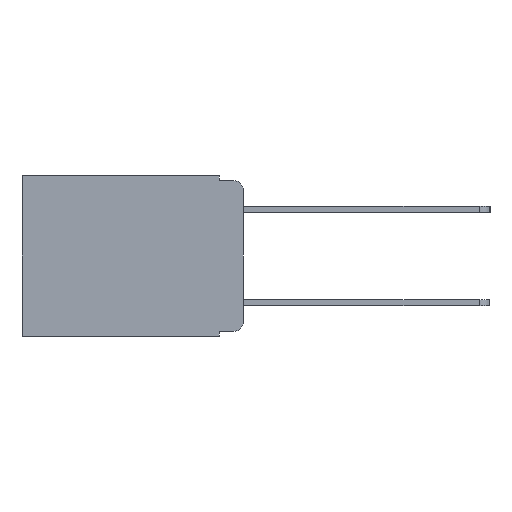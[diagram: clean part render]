
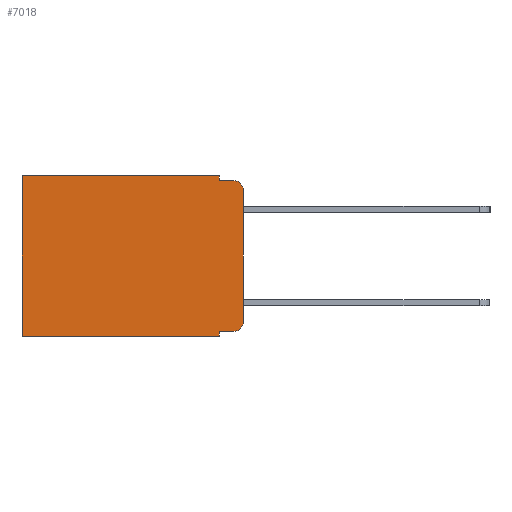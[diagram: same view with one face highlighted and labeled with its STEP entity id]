
A CAD part, left-side view. The second image highlights one B-rep face of the part: STEP entity #7018.
In plain terms, the highlighted planar face has unit normal (-1, 0, 0).
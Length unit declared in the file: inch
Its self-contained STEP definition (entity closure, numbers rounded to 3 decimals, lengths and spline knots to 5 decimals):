
#772 = CARTESIAN_POINT ( 'NONE',  ( 0.298, 0.473, 0. ) ) ;
#1231 = VERTEX_POINT ( 'NONE', #13358 ) ;
#1259 = ORIENTED_EDGE ( 'NONE', *, *, #11092, .T. ) ;
#1486 = DIRECTION ( 'NONE',  ( 0., 0., -1. ) ) ;
#1542 = VERTEX_POINT ( 'NONE', #14407 ) ;
#2212 = VECTOR ( 'NONE', #12062, 39.37008 ) ;
#2250 = VERTEX_POINT ( 'NONE', #7508 ) ;
#2955 = LINE ( 'NONE', #7042, #14989 ) ;
#3022 = CARTESIAN_POINT ( 'NONE',  ( 0.298, 0.02, -0.03 ) ) ;
#3057 = ORIENTED_EDGE ( 'NONE', *, *, #14924, .F. ) ;
#3107 = CARTESIAN_POINT ( 'NONE',  ( 0.298, 0.051, -0.333 ) ) ;
#3242 = CARTESIAN_POINT ( 'NONE',  ( 0.298, 0., -0.03 ) ) ;
#3285 = ORIENTED_EDGE ( 'NONE', *, *, #13959, .F. ) ;
#3559 = LINE ( 'NONE', #6247, #11307 ) ;
#3753 = VERTEX_POINT ( 'NONE', #772 ) ;
#3940 = ORIENTED_EDGE ( 'NONE', *, *, #17739, .F. ) ;
#4018 = CARTESIAN_POINT ( 'NONE',  ( 0.298, 0.051, -0.343 ) ) ;
#4378 = CARTESIAN_POINT ( 'NONE',  ( 0.298, 0.051, 0. ) ) ;
#4478 = VERTEX_POINT ( 'NONE', #18992 ) ;
#4552 = DIRECTION ( 'NONE',  ( 0., 0., -1. ) ) ;
#4741 = CARTESIAN_POINT ( 'NONE',  ( 0.298, 0., 0. ) ) ;
#4965 = VECTOR ( 'NONE', #14469, 39.37008 ) ;
#5462 = AXIS2_PLACEMENT_3D ( 'NONE', #3022, #13197, #4552 ) ;
#5633 = LINE ( 'NONE', #10392, #11926 ) ;
#5701 = DIRECTION ( 'NONE',  ( 0., 0., -1. ) ) ;
#5858 = AXIS2_PLACEMENT_3D ( 'NONE', #8838, #18699, #10257 ) ;
#5867 = ORIENTED_EDGE ( 'NONE', *, *, #13007, .T. ) ;
#6245 = VECTOR ( 'NONE', #8428, 39.37008 ) ;
#6247 = CARTESIAN_POINT ( 'NONE',  ( 0.298, 0.051, -0.333 ) ) ;
#6334 = EDGE_LOOP ( 'NONE', ( #3940, #13733, #3057, #3285, #7692, #5867, #6750, #8131, #1259, #7195 ) ) ;
#6578 = DIRECTION ( 'NONE',  ( 0., 0., -1. ) ) ;
#6650 = LINE ( 'NONE', #13564, #2212 ) ;
#6750 = ORIENTED_EDGE ( 'NONE', *, *, #17389, .F. ) ;
#7018 = ADVANCED_FACE ( 'NONE', ( #14549 ), #16247, .F. ) ;
#7042 = CARTESIAN_POINT ( 'NONE',  ( 0.298, 0., 0. ) ) ;
#7195 = ORIENTED_EDGE ( 'NONE', *, *, #10144, .T. ) ;
#7508 = CARTESIAN_POINT ( 'NONE',  ( 0.298, 0.02, -0.333 ) ) ;
#7692 = ORIENTED_EDGE ( 'NONE', *, *, #8380, .T. ) ;
#7841 = DIRECTION ( 'NONE',  ( 0., 1., 0. ) ) ;
#8131 = ORIENTED_EDGE ( 'NONE', *, *, #12046, .F. ) ;
#8380 = EDGE_CURVE ( 'NONE', #1542, #3753, #6650, .T. ) ;
#8428 = DIRECTION ( 'NONE',  ( 0., -1., 0. ) ) ;
#8658 = CIRCLE ( 'NONE', #5858, 0.02 ) ;
#8838 = CARTESIAN_POINT ( 'NONE',  ( 0.298, 0.02, -0.313 ) ) ;
#8944 = VERTEX_POINT ( 'NONE', #16428 ) ;
#9291 = LINE ( 'NONE', #4378, #4965 ) ;
#9412 = VERTEX_POINT ( 'NONE', #3107 ) ;
#9505 = VERTEX_POINT ( 'NONE', #3242 ) ;
#9665 = LINE ( 'NONE', #18315, #6245 ) ;
#10001 = CARTESIAN_POINT ( 'NONE',  ( 0.298, 0.051, 0. ) ) ;
#10144 = EDGE_CURVE ( 'NONE', #2250, #4478, #8658, .T. ) ;
#10257 = DIRECTION ( 'NONE',  ( 0., 0., -1. ) ) ;
#10392 = CARTESIAN_POINT ( 'NONE',  ( 0.298, 0.473, 0. ) ) ;
#11092 = EDGE_CURVE ( 'NONE', #9412, #2250, #3559, .T. ) ;
#11307 = VECTOR ( 'NONE', #16299, 39.37008 ) ;
#11420 = LINE ( 'NONE', #13589, #11869 ) ;
#11435 = LINE ( 'NONE', #10001, #18475 ) ;
#11869 = VECTOR ( 'NONE', #7841, 39.37008 ) ;
#11926 = VECTOR ( 'NONE', #1486, 39.37008 ) ;
#12046 = EDGE_CURVE ( 'NONE', #9412, #17710, #9291, .T. ) ;
#12062 = DIRECTION ( 'NONE',  ( 0., 1., 0. ) ) ;
#12100 = VERTEX_POINT ( 'NONE', #18660 ) ;
#13007 = EDGE_CURVE ( 'NONE', #3753, #12100, #5633, .T. ) ;
#13197 = DIRECTION ( 'NONE',  ( -1., 0., 0. ) ) ;
#13358 = CARTESIAN_POINT ( 'NONE',  ( 0.298, 0.051, -0.01 ) ) ;
#13564 = CARTESIAN_POINT ( 'NONE',  ( 0.298, 0., 0. ) ) ;
#13589 = CARTESIAN_POINT ( 'NONE',  ( 0.298, 0., -0.343 ) ) ;
#13733 = ORIENTED_EDGE ( 'NONE', *, *, #15891, .T. ) ;
#13959 = EDGE_CURVE ( 'NONE', #1542, #1231, #11435, .T. ) ;
#14407 = CARTESIAN_POINT ( 'NONE',  ( 0.298, 0.051, 0. ) ) ;
#14469 = DIRECTION ( 'NONE',  ( 0., 0., -1. ) ) ;
#14549 = FACE_OUTER_BOUND ( 'NONE', #6334, .T. ) ;
#14556 = DIRECTION ( 'NONE',  ( 1., 0., 0. ) ) ;
#14924 = EDGE_CURVE ( 'NONE', #1231, #8944, #9665, .T. ) ;
#14989 = VECTOR ( 'NONE', #17052, 39.37008 ) ;
#15063 = CIRCLE ( 'NONE', #5462, 0.02 ) ;
#15891 = EDGE_CURVE ( 'NONE', #9505, #8944, #15063, .T. ) ;
#16247 = PLANE ( 'NONE',  #18658 ) ;
#16299 = DIRECTION ( 'NONE',  ( 0., -1., 0. ) ) ;
#16428 = CARTESIAN_POINT ( 'NONE',  ( 0.298, 0.02, -0.01 ) ) ;
#17052 = DIRECTION ( 'NONE',  ( 0., 0., -1. ) ) ;
#17389 = EDGE_CURVE ( 'NONE', #17710, #12100, #11420, .T. ) ;
#17710 = VERTEX_POINT ( 'NONE', #4018 ) ;
#17739 = EDGE_CURVE ( 'NONE', #9505, #4478, #2955, .T. ) ;
#18315 = CARTESIAN_POINT ( 'NONE',  ( 0.298, 0.051, -0.01 ) ) ;
#18475 = VECTOR ( 'NONE', #5701, 39.37008 ) ;
#18658 = AXIS2_PLACEMENT_3D ( 'NONE', #4741, #14556, #6578 ) ;
#18660 = CARTESIAN_POINT ( 'NONE',  ( 0.298, 0.473, -0.343 ) ) ;
#18699 = DIRECTION ( 'NONE',  ( -1., 0., 0. ) ) ;
#18992 = CARTESIAN_POINT ( 'NONE',  ( 0.298, 0., -0.313 ) ) ;
